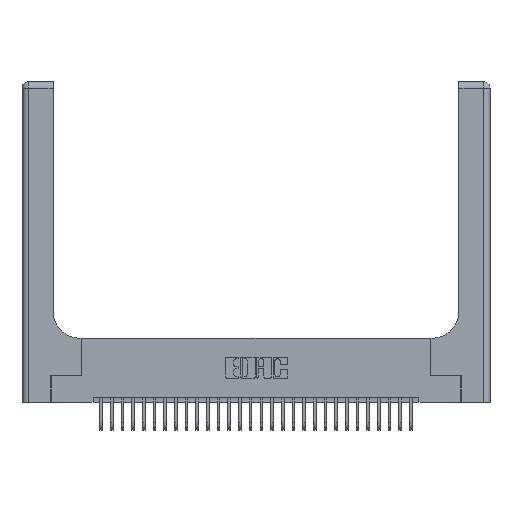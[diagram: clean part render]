
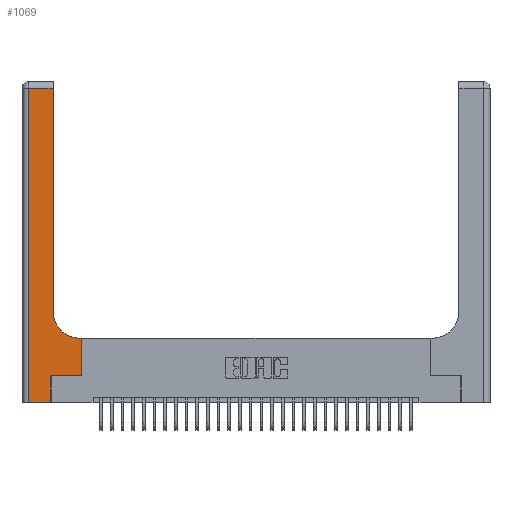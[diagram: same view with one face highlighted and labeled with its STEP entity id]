
A CAD part, top view. The second image highlights one B-rep face of the part: STEP entity #1069.
In plain terms, the highlighted planar face has unit normal (0, 0, 1).
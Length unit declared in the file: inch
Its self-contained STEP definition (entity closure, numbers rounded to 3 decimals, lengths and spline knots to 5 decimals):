
#69 = ORIENTED_EDGE ( 'NONE', *, *, #17449, .T. ) ;
#164 = CARTESIAN_POINT ( 'NONE',  ( 0., 2.94, 0.37 ) ) ;
#251 = EDGE_CURVE ( 'NONE', #25590, #31034, #6731, .T. ) ;
#819 = CIRCLE ( 'NONE', #4069, 0.25 ) ;
#1069 = ADVANCED_FACE ( 'NONE', ( #21194 ), #7522, .F. ) ;
#1145 = CARTESIAN_POINT ( 'NONE',  ( 0.2915, 0.6, 0.37 ) ) ;
#1803 = LINE ( 'NONE', #20495, #20366 ) ;
#2449 = LINE ( 'NONE', #15794, #24549 ) ;
#3050 = LINE ( 'NONE', #20862, #18141 ) ;
#4069 = AXIS2_PLACEMENT_3D ( 'NONE', #23982, #31721, #4568 ) ;
#4290 = CARTESIAN_POINT ( 'NONE',  ( 0.06, 0., 0.37 ) ) ;
#4388 = DIRECTION ( 'NONE',  ( 1., 0., 0. ) ) ;
#4428 = ORIENTED_EDGE ( 'NONE', *, *, #25062, .T. ) ;
#4568 = DIRECTION ( 'NONE',  ( 1., 0., 0. ) ) ;
#5257 = CARTESIAN_POINT ( 'NONE',  ( 0., 3., 0.37 ) ) ;
#5279 = EDGE_CURVE ( 'NONE', #16847, #10323, #7800, .T. ) ;
#6165 = CARTESIAN_POINT ( 'NONE',  ( 0.5585, 0.25, 0.37 ) ) ;
#6731 = LINE ( 'NONE', #164, #25741 ) ;
#6924 = CARTESIAN_POINT ( 'NONE',  ( 0.269, 0., 0.37 ) ) ;
#7522 = PLANE ( 'NONE',  #19436 ) ;
#7800 = LINE ( 'NONE', #18422, #12463 ) ;
#8927 = EDGE_CURVE ( 'NONE', #10323, #24762, #16656, .T. ) ;
#9248 = DIRECTION ( 'NONE',  ( 1., 0., 0. ) ) ;
#9467 = CARTESIAN_POINT ( 'NONE',  ( 0., 0., 0.37 ) ) ;
#9935 = VECTOR ( 'NONE', #9248, 39.37008 ) ;
#10323 = VERTEX_POINT ( 'NONE', #23478 ) ;
#11130 = LINE ( 'NONE', #9467, #9935 ) ;
#11388 = DIRECTION ( 'NONE',  ( 0., 1., 0. ) ) ;
#11511 = EDGE_CURVE ( 'NONE', #26804, #13839, #11130, .T. ) ;
#12463 = VECTOR ( 'NONE', #11388, 39.37008 ) ;
#12504 = ORIENTED_EDGE ( 'NONE', *, *, #18071, .T. ) ;
#12631 = DIRECTION ( 'NONE',  ( 0., 0., -1. ) ) ;
#13839 = VERTEX_POINT ( 'NONE', #6924 ) ;
#15342 = DIRECTION ( 'NONE',  ( -1., 0., 0. ) ) ;
#15794 = CARTESIAN_POINT ( 'NONE',  ( 0.269, 0., 0.37 ) ) ;
#15902 = EDGE_CURVE ( 'NONE', #27577, #25590, #1803, .T. ) ;
#16656 = LINE ( 'NONE', #1145, #28648 ) ;
#16737 = EDGE_LOOP ( 'NONE', ( #27940, #18705, #4428, #17541, #69, #12504, #31837, #24311, #28687 ) ) ;
#16738 = VECTOR ( 'NONE', #4388, 39.37008 ) ;
#16847 = VERTEX_POINT ( 'NONE', #6165 ) ;
#17449 = EDGE_CURVE ( 'NONE', #13839, #31971, #2449, .T. ) ;
#17476 = DIRECTION ( 'NONE',  ( -1., 0., 0. ) ) ;
#17541 = ORIENTED_EDGE ( 'NONE', *, *, #11511, .T. ) ;
#17571 = CARTESIAN_POINT ( 'NONE',  ( 0.06, 2.94, 0.37 ) ) ;
#18071 = EDGE_CURVE ( 'NONE', #31971, #16847, #18283, .T. ) ;
#18141 = VECTOR ( 'NONE', #25658, 39.37008 ) ;
#18275 = DIRECTION ( 'NONE',  ( 0., 1., 0. ) ) ;
#18283 = LINE ( 'NONE', #22147, #16738 ) ;
#18422 = CARTESIAN_POINT ( 'NONE',  ( 0.5585, 0.25, 0.37 ) ) ;
#18705 = ORIENTED_EDGE ( 'NONE', *, *, #251, .T. ) ;
#19310 = CARTESIAN_POINT ( 'NONE',  ( 0.2915, 0.85, 0.37 ) ) ;
#19436 = AXIS2_PLACEMENT_3D ( 'NONE', #5257, #12631, #15342 ) ;
#20366 = VECTOR ( 'NONE', #22903, 39.37008 ) ;
#20495 = CARTESIAN_POINT ( 'NONE',  ( 0.2915, 3., 0.37 ) ) ;
#20862 = CARTESIAN_POINT ( 'NONE',  ( 0.06, 3., 0.37 ) ) ;
#21194 = FACE_OUTER_BOUND ( 'NONE', #16737, .T. ) ;
#22147 = CARTESIAN_POINT ( 'NONE',  ( 0.269, 0.25, 0.37 ) ) ;
#22788 = CARTESIAN_POINT ( 'NONE',  ( 0.2915, 2.94, 0.37 ) ) ;
#22903 = DIRECTION ( 'NONE',  ( 0., 1., 0. ) ) ;
#23478 = CARTESIAN_POINT ( 'NONE',  ( 0.5585, 0.6, 0.37 ) ) ;
#23982 = CARTESIAN_POINT ( 'NONE',  ( 0.5415, 0.85, 0.37 ) ) ;
#24021 = EDGE_CURVE ( 'NONE', #24762, #27577, #819, .T. ) ;
#24311 = ORIENTED_EDGE ( 'NONE', *, *, #8927, .T. ) ;
#24549 = VECTOR ( 'NONE', #18275, 39.37008 ) ;
#24762 = VERTEX_POINT ( 'NONE', #29104 ) ;
#24982 = DIRECTION ( 'NONE',  ( -1., 0., 0. ) ) ;
#25062 = EDGE_CURVE ( 'NONE', #31034, #26804, #3050, .T. ) ;
#25590 = VERTEX_POINT ( 'NONE', #22788 ) ;
#25658 = DIRECTION ( 'NONE',  ( 0., -1., 0. ) ) ;
#25741 = VECTOR ( 'NONE', #17476, 39.37008 ) ;
#25774 = CARTESIAN_POINT ( 'NONE',  ( 0.269, 0.25, 0.37 ) ) ;
#26804 = VERTEX_POINT ( 'NONE', #4290 ) ;
#27577 = VERTEX_POINT ( 'NONE', #19310 ) ;
#27940 = ORIENTED_EDGE ( 'NONE', *, *, #15902, .T. ) ;
#28648 = VECTOR ( 'NONE', #24982, 39.37008 ) ;
#28687 = ORIENTED_EDGE ( 'NONE', *, *, #24021, .T. ) ;
#29104 = CARTESIAN_POINT ( 'NONE',  ( 0.5415, 0.6, 0.37 ) ) ;
#31034 = VERTEX_POINT ( 'NONE', #17571 ) ;
#31721 = DIRECTION ( 'NONE',  ( 0., 0., -1. ) ) ;
#31837 = ORIENTED_EDGE ( 'NONE', *, *, #5279, .T. ) ;
#31971 = VERTEX_POINT ( 'NONE', #25774 ) ;
